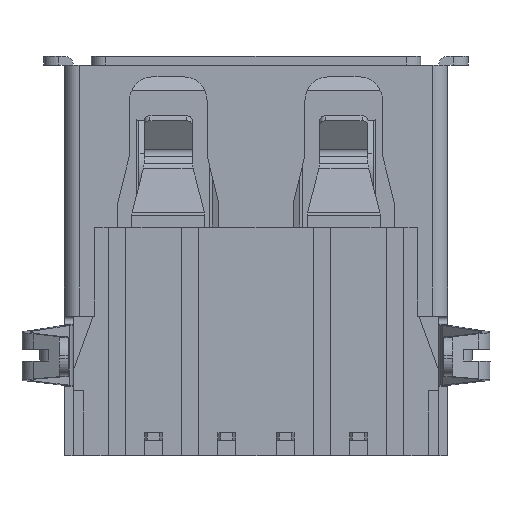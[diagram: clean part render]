
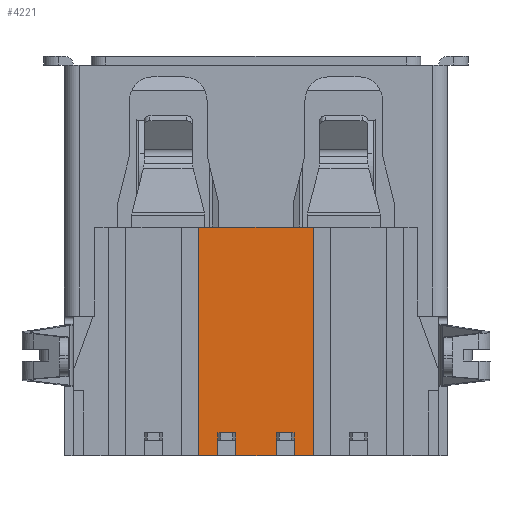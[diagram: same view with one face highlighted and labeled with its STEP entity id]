
A CAD part, front view. The second image highlights one B-rep face of the part: STEP entity #4221.
In plain terms, the highlighted planar face has unit normal (0, -1, 0).
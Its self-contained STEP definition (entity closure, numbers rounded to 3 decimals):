
#483 = VERTEX_POINT ( 'NONE', #2893 ) ;
#507 = LINE ( 'NONE', #3987, #18493 ) ;
#856 = ORIENTED_EDGE ( 'NONE', *, *, #10950, .T. ) ;
#1239 = CARTESIAN_POINT ( 'NONE',  ( -3.03, -6.1, 8.2 ) ) ;
#1327 = CARTESIAN_POINT ( 'NONE',  ( 3.99, -6.1, 6.95 ) ) ;
#1907 = FACE_OUTER_BOUND ( 'NONE', #2996, .T. ) ;
#1950 = ORIENTED_EDGE ( 'NONE', *, *, #3802, .T. ) ;
#1964 = DIRECTION ( 'NONE',  ( 1., 0., 0. ) ) ;
#1982 = EDGE_CURVE ( 'NONE', #20634, #12668, #17857, .T. ) ;
#2288 = VERTEX_POINT ( 'NONE', #1327 ) ;
#2392 = CARTESIAN_POINT ( 'NONE',  ( 0., -6.1, 8.2 ) ) ;
#2576 = VERTEX_POINT ( 'NONE', #17905 ) ;
#2581 = LINE ( 'NONE', #16257, #18853 ) ;
#2672 = CARTESIAN_POINT ( 'NONE',  ( 3.99, -6.1, 5.55 ) ) ;
#2893 = CARTESIAN_POINT ( 'NONE',  ( -3.03, -6.1, 4.3 ) ) ;
#2996 = EDGE_LOOP ( 'NONE', ( #6896, #17149, #20410, #8398, #7672, #14240, #856, #20454, #16011, #1950, #7102, #20854 ) ) ;
#3250 = CARTESIAN_POINT ( 'NONE',  ( 3.99, -6.1, 0. ) ) ;
#3802 = EDGE_CURVE ( 'NONE', #22138, #12705, #11495, .T. ) ;
#3987 = CARTESIAN_POINT ( 'NONE',  ( 4.77, -6.1, 0. ) ) ;
#4002 = CARTESIAN_POINT ( 'NONE',  ( 4.77, -6.1, 4.95 ) ) ;
#4150 = EDGE_CURVE ( 'NONE', #12705, #14721, #11469, .T. ) ;
#4221 = ADVANCED_FACE ( 'NONE', ( #1907 ), #20420, .T. ) ;
#4422 = DIRECTION ( 'NONE',  ( 0., 0., 1. ) ) ;
#4760 = VERTEX_POINT ( 'NONE', #15016 ) ;
#4940 = CARTESIAN_POINT ( 'NONE',  ( 0., -6.1, 0. ) ) ;
#5653 = DIRECTION ( 'NONE',  ( 0., 0., -1. ) ) ;
#6322 = CARTESIAN_POINT ( 'NONE',  ( 4.77, -6.1, 4.95 ) ) ;
#6403 = CARTESIAN_POINT ( 'NONE',  ( 3.99, -6.1, 5.55 ) ) ;
#6698 = LINE ( 'NONE', #18816, #21140 ) ;
#6896 = ORIENTED_EDGE ( 'NONE', *, *, #7284, .T. ) ;
#7102 = ORIENTED_EDGE ( 'NONE', *, *, #4150, .T. ) ;
#7284 = EDGE_CURVE ( 'NONE', #2576, #2288, #15248, .T. ) ;
#7362 = DIRECTION ( 'NONE',  ( -1., 0., 0. ) ) ;
#7612 = DIRECTION ( 'NONE',  ( 0., 0., -1. ) ) ;
#7672 = ORIENTED_EDGE ( 'NONE', *, *, #8823, .T. ) ;
#7994 = VERTEX_POINT ( 'NONE', #1239 ) ;
#8398 = ORIENTED_EDGE ( 'NONE', *, *, #9700, .F. ) ;
#8473 = LINE ( 'NONE', #15184, #12091 ) ;
#8647 = VECTOR ( 'NONE', #4422, 1000. ) ;
#8823 = EDGE_CURVE ( 'NONE', #19379, #7994, #17879, .T. ) ;
#9562 = DIRECTION ( 'NONE',  ( 1., 0., 0. ) ) ;
#9700 = EDGE_CURVE ( 'NONE', #19379, #12668, #12881, .T. ) ;
#9878 = VECTOR ( 'NONE', #7612, 1000. ) ;
#10544 = EDGE_CURVE ( 'NONE', #2576, #14721, #507, .T. ) ;
#10950 = EDGE_CURVE ( 'NONE', #483, #4760, #2581, .T. ) ;
#11276 = VECTOR ( 'NONE', #19557, 1000. ) ;
#11323 = CARTESIAN_POINT ( 'NONE',  ( 4.77, -6.1, 7.55 ) ) ;
#11336 = LINE ( 'NONE', #3250, #15194 ) ;
#11469 = LINE ( 'NONE', #6403, #17250 ) ;
#11495 = LINE ( 'NONE', #18336, #8647 ) ;
#12091 = VECTOR ( 'NONE', #20568, 1000. ) ;
#12103 = DIRECTION ( 'NONE',  ( 0., -1., 0. ) ) ;
#12658 = DIRECTION ( 'NONE',  ( 1., 0., 0. ) ) ;
#12668 = VERTEX_POINT ( 'NONE', #11323 ) ;
#12705 = VERTEX_POINT ( 'NONE', #2672 ) ;
#12736 = CARTESIAN_POINT ( 'NONE',  ( 3.99, -6.1, 7.55 ) ) ;
#12881 = LINE ( 'NONE', #21647, #9878 ) ;
#13276 = EDGE_CURVE ( 'NONE', #483, #7994, #8473, .T. ) ;
#13839 = CARTESIAN_POINT ( 'NONE',  ( 3.99, -6.1, 7.55 ) ) ;
#14093 = CARTESIAN_POINT ( 'NONE',  ( 4.77, -6.1, 8.2 ) ) ;
#14201 = LINE ( 'NONE', #4002, #19743 ) ;
#14229 = EDGE_CURVE ( 'NONE', #2288, #20634, #11336, .T. ) ;
#14240 = ORIENTED_EDGE ( 'NONE', *, *, #13276, .F. ) ;
#14721 = VERTEX_POINT ( 'NONE', #19212 ) ;
#15016 = CARTESIAN_POINT ( 'NONE',  ( 4.77, -6.1, 4.3 ) ) ;
#15184 = CARTESIAN_POINT ( 'NONE',  ( -3.03, -6.1, 0. ) ) ;
#15194 = VECTOR ( 'NONE', #16922, 1000. ) ;
#15248 = LINE ( 'NONE', #18521, #17295 ) ;
#15801 = AXIS2_PLACEMENT_3D ( 'NONE', #4940, #12103, #20311 ) ;
#16011 = ORIENTED_EDGE ( 'NONE', *, *, #18199, .T. ) ;
#16257 = CARTESIAN_POINT ( 'NONE',  ( 0., -6.1, 4.3 ) ) ;
#16922 = DIRECTION ( 'NONE',  ( 0., 0., 1. ) ) ;
#17047 = DIRECTION ( 'NONE',  ( -1., 0., 0. ) ) ;
#17149 = ORIENTED_EDGE ( 'NONE', *, *, #14229, .T. ) ;
#17250 = VECTOR ( 'NONE', #9562, 1000. ) ;
#17295 = VECTOR ( 'NONE', #17047, 1000. ) ;
#17857 = LINE ( 'NONE', #13839, #19647 ) ;
#17879 = LINE ( 'NONE', #2392, #11276 ) ;
#17905 = CARTESIAN_POINT ( 'NONE',  ( 4.77, -6.1, 6.95 ) ) ;
#18197 = CARTESIAN_POINT ( 'NONE',  ( 3.99, -6.1, 4.95 ) ) ;
#18199 = EDGE_CURVE ( 'NONE', #21808, #22138, #14201, .T. ) ;
#18336 = CARTESIAN_POINT ( 'NONE',  ( 3.99, -6.1, 0. ) ) ;
#18493 = VECTOR ( 'NONE', #5653, 1000. ) ;
#18521 = CARTESIAN_POINT ( 'NONE',  ( 4.77, -6.1, 6.95 ) ) ;
#18816 = CARTESIAN_POINT ( 'NONE',  ( 4.77, -6.1, 0. ) ) ;
#18853 = VECTOR ( 'NONE', #12658, 1000. ) ;
#19212 = CARTESIAN_POINT ( 'NONE',  ( 4.77, -6.1, 5.55 ) ) ;
#19379 = VERTEX_POINT ( 'NONE', #14093 ) ;
#19557 = DIRECTION ( 'NONE',  ( -1., 0., 0. ) ) ;
#19647 = VECTOR ( 'NONE', #1964, 1000. ) ;
#19743 = VECTOR ( 'NONE', #7362, 1000. ) ;
#20311 = DIRECTION ( 'NONE',  ( 0., 0., -1. ) ) ;
#20389 = DIRECTION ( 'NONE',  ( 0., 0., -1. ) ) ;
#20410 = ORIENTED_EDGE ( 'NONE', *, *, #1982, .T. ) ;
#20420 = PLANE ( 'NONE',  #15801 ) ;
#20454 = ORIENTED_EDGE ( 'NONE', *, *, #21251, .F. ) ;
#20568 = DIRECTION ( 'NONE',  ( 0., 0., 1. ) ) ;
#20634 = VERTEX_POINT ( 'NONE', #12736 ) ;
#20854 = ORIENTED_EDGE ( 'NONE', *, *, #10544, .F. ) ;
#21140 = VECTOR ( 'NONE', #20389, 1000. ) ;
#21251 = EDGE_CURVE ( 'NONE', #21808, #4760, #6698, .T. ) ;
#21647 = CARTESIAN_POINT ( 'NONE',  ( 4.77, -6.1, 0. ) ) ;
#21808 = VERTEX_POINT ( 'NONE', #6322 ) ;
#22138 = VERTEX_POINT ( 'NONE', #18197 ) ;
